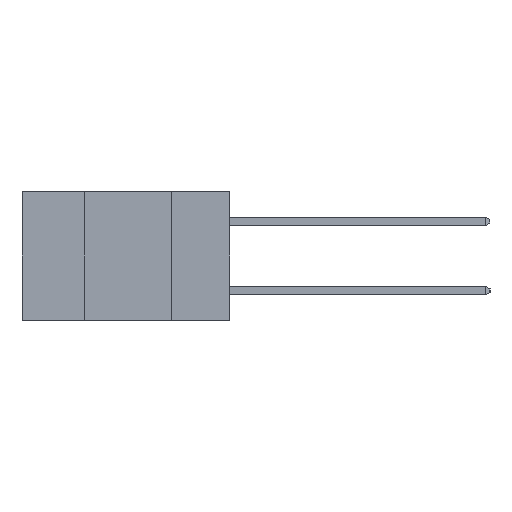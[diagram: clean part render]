
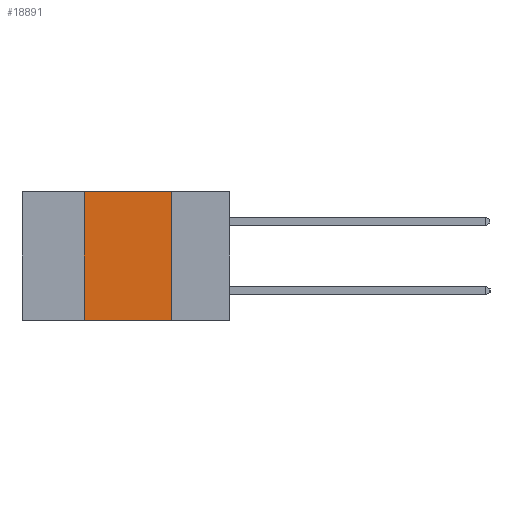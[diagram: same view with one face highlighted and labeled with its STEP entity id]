
A CAD part, left-side view. The second image highlights one B-rep face of the part: STEP entity #18891.
In plain terms, the highlighted planar face has unit normal (-1, 0, 0).
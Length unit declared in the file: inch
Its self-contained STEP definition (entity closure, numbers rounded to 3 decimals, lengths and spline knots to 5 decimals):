
#293 = ORIENTED_EDGE ( 'NONE', *, *, #10129, .F. ) ;
#1082 = CARTESIAN_POINT ( 'NONE',  ( 0., 0.42, 0. ) ) ;
#1174 = FACE_OUTER_BOUND ( 'NONE', #1742, .T. ) ;
#1285 = ORIENTED_EDGE ( 'NONE', *, *, #9602, .F. ) ;
#1742 = EDGE_LOOP ( 'NONE', ( #293, #3298, #1285, #9355 ) ) ;
#2485 = CARTESIAN_POINT ( 'NONE',  ( 0., 0.17, -0.37 ) ) ;
#2750 = VERTEX_POINT ( 'NONE', #12359 ) ;
#3298 = ORIENTED_EDGE ( 'NONE', *, *, #18915, .F. ) ;
#3381 = CARTESIAN_POINT ( 'NONE',  ( 0., 0.42, -0.37 ) ) ;
#4675 = CARTESIAN_POINT ( 'NONE',  ( 0., 0.6, 0. ) ) ;
#5436 = LINE ( 'NONE', #11081, #13538 ) ;
#5444 = LINE ( 'NONE', #4675, #17142 ) ;
#7884 = CARTESIAN_POINT ( 'NONE',  ( 0., 0.6, 0. ) ) ;
#7980 = LINE ( 'NONE', #18561, #20009 ) ;
#9355 = ORIENTED_EDGE ( 'NONE', *, *, #9444, .T. ) ;
#9444 = EDGE_CURVE ( 'NONE', #16681, #16277, #7980, .T. ) ;
#9602 = EDGE_CURVE ( 'NONE', #16681, #10579, #5436, .T. ) ;
#10129 = EDGE_CURVE ( 'NONE', #2750, #16277, #16167, .T. ) ;
#10579 = VERTEX_POINT ( 'NONE', #1082 ) ;
#10943 = AXIS2_PLACEMENT_3D ( 'NONE', #7884, #20407, #11129 ) ;
#11081 = CARTESIAN_POINT ( 'NONE',  ( 0., 0.42, -0.37 ) ) ;
#11129 = DIRECTION ( 'NONE',  ( 0., 0., -1. ) ) ;
#11448 = DIRECTION ( 'NONE',  ( 0., 0., -1. ) ) ;
#11639 = DIRECTION ( 'NONE',  ( 0., 0., 1. ) ) ;
#11664 = CARTESIAN_POINT ( 'NONE',  ( 0., 0.17, -0.37 ) ) ;
#12359 = CARTESIAN_POINT ( 'NONE',  ( 0., 0.17, 0. ) ) ;
#13538 = VECTOR ( 'NONE', #11639, 39.37008 ) ;
#16167 = LINE ( 'NONE', #11664, #19744 ) ;
#16277 = VERTEX_POINT ( 'NONE', #2485 ) ;
#16681 = VERTEX_POINT ( 'NONE', #3381 ) ;
#17142 = VECTOR ( 'NONE', #17418, 39.37008 ) ;
#17418 = DIRECTION ( 'NONE',  ( 0., -1., 0. ) ) ;
#18123 = DIRECTION ( 'NONE',  ( 0., -1., 0. ) ) ;
#18561 = CARTESIAN_POINT ( 'NONE',  ( 0., 0.6, -0.37 ) ) ;
#18888 = PLANE ( 'NONE',  #10943 ) ;
#18891 = ADVANCED_FACE ( 'NONE', ( #1174 ), #18888, .F. ) ;
#18915 = EDGE_CURVE ( 'NONE', #10579, #2750, #5444, .T. ) ;
#19744 = VECTOR ( 'NONE', #11448, 39.37008 ) ;
#20009 = VECTOR ( 'NONE', #18123, 39.37008 ) ;
#20407 = DIRECTION ( 'NONE',  ( 1., 0., 0. ) ) ;
